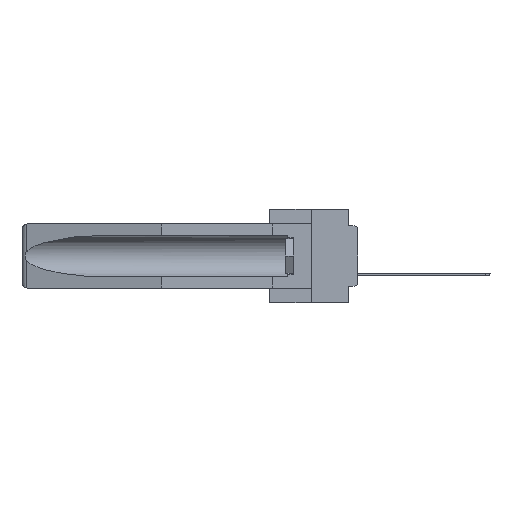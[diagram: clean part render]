
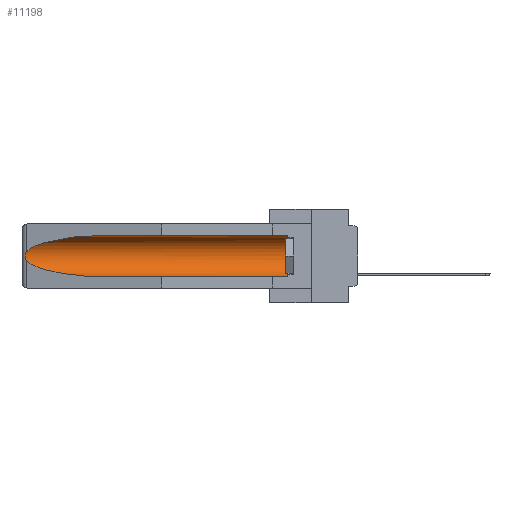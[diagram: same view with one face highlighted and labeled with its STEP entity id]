
A CAD part, left-side view. The second image highlights one B-rep face of the part: STEP entity #11198.
In plain terms, the highlighted cylindrical face has radius 2.857 mm (diameter 5.715 mm), a partial arc.
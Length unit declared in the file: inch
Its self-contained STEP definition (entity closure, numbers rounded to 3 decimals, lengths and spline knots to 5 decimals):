
#1793 = CIRCLE ( 'NONE', #25780, 0.1125 ) ;
#2804 = EDGE_CURVE ( 'NONE', #11947, #5407, #24546, .T. ) ;
#2918 = CARTESIAN_POINT ( 'NONE',  ( 0.26597, 1.52961, -0.15275 ) ) ;
#3536 = VECTOR ( 'NONE', #25333, 39.37008 ) ;
#3707 = CARTESIAN_POINT ( 'NONE',  ( 0.155, -0.30754, -0.1715 ) ) ;
#4063 = DIRECTION ( 'NONE',  ( 0., 1., 0. ) ) ;
#4702 = VERTEX_POINT ( 'NONE', #28749 ) ;
#5165 = VERTEX_POINT ( 'NONE', #16632 ) ;
#5407 = VERTEX_POINT ( 'NONE', #25781 ) ;
#5411 = CARTESIAN_POINT ( 'NONE',  ( 0.2675, 1.53308, -0.17534 ) ) ;
#5635 = CARTESIAN_POINT ( 'NONE',  ( 0.26597, 1.5296, -0.19026 ) ) ;
#5731 = CARTESIAN_POINT ( 'NONE',  ( 0.26537, 1.52718, -0.19328 ) ) ;
#7159 = LINE ( 'NONE', #12648, #3536 ) ;
#7700 = EDGE_CURVE ( 'NONE', #5165, #10313, #9998, .T. ) ;
#8202 = ORIENTED_EDGE ( 'NONE', *, *, #21001, .T. ) ;
#8883 = VECTOR ( 'NONE', #31061, 39.37008 ) ;
#9124 = AXIS2_PLACEMENT_3D ( 'NONE', #3707, #4063, #14493 ) ;
#9139 = CARTESIAN_POINT ( 'NONE',  ( 0.26537, 1.52718, -0.14972 ) ) ;
#9626 = EDGE_CURVE ( 'NONE', #10486, #11947, #1793, .T. ) ;
#9998 =( BOUNDED_CURVE ( )  B_SPLINE_CURVE ( 3, ( #27462, #22302, #32775, #30266 ),
 .UNSPECIFIED., .F., .F. ) 
 B_SPLINE_CURVE_WITH_KNOTS ( ( 4, 4 ),
 ( 0.1948, 1.5708 ),
 .UNSPECIFIED. ) 
 CURVE ( )  GEOMETRIC_REPRESENTATION_ITEM ( )  RATIONAL_B_SPLINE_CURVE ( ( 1., 0.848, 0.848, 1. ) ) 
 REPRESENTATION_ITEM ( '' )  );
#10286 = ORIENTED_EDGE ( 'NONE', *, *, #9626, .T. ) ;
#10313 = VERTEX_POINT ( 'NONE', #30845 ) ;
#10486 = VERTEX_POINT ( 'NONE', #29428 ) ;
#10651 = CARTESIAN_POINT ( 'NONE',  ( 0.2673, 1.53269, -0.17917 ) ) ;
#10661 = EDGE_LOOP ( 'NONE', ( #23231, #8202, #16517, #16245, #10286, #27308 ) ) ;
#10835 = FACE_OUTER_BOUND ( 'NONE', #10661, .T. ) ;
#11137 = CARTESIAN_POINT ( 'NONE',  ( 0.25451, 1.48313, -0.09465 ) ) ;
#11198 = ADVANCED_FACE ( 'NONE', ( #10835 ), #18476, .F. ) ;
#11947 = VERTEX_POINT ( 'NONE', #14923 ) ;
#12648 = CARTESIAN_POINT ( 'NONE',  ( 0.155, -0.30754, -0.284 ) ) ;
#13074 = CARTESIAN_POINT ( 'NONE',  ( 0.155, -0.30754, -0.059 ) ) ;
#14493 = DIRECTION ( 'NONE',  ( 0., 0., 1. ) ) ;
#14923 = CARTESIAN_POINT ( 'NONE',  ( 0.155, 0.126, -0.059 ) ) ;
#16245 = ORIENTED_EDGE ( 'NONE', *, *, #21391, .F. ) ;
#16517 = ORIENTED_EDGE ( 'NONE', *, *, #7700, .T. ) ;
#16632 = CARTESIAN_POINT ( 'NONE',  ( 0.26537, 1.52718, -0.19328 ) ) ;
#18269 = CARTESIAN_POINT ( 'NONE',  ( 0.26655, 1.53094, -0.18657 ) ) ;
#18476 = CYLINDRICAL_SURFACE ( 'NONE', #9124, 0.1125 ) ;
#18505 = CARTESIAN_POINT ( 'NONE',  ( 0.26654, 1.53092, -0.15636 ) ) ;
#19016 = B_SPLINE_CURVE_WITH_KNOTS ( 'NONE', 3,
 ( #31439, #2918, #18505, #28531, #21087, #5411, #10651, #18269, #5635, #5731 ),
 .UNSPECIFIED., .F., .F.,
 ( 4, 2, 2, 2, 4 ),
 ( 0., 0.00029, 0.00058, 0.00087, 0.00117 ),
 .UNSPECIFIED. ) ;
#21001 = EDGE_CURVE ( 'NONE', #4702, #5165, #19016, .T. ) ;
#21087 = CARTESIAN_POINT ( 'NONE',  ( 0.2675, 1.53308, -0.16763 ) ) ;
#21391 = EDGE_CURVE ( 'NONE', #10486, #10313, #7159, .T. ) ;
#21472 = CARTESIAN_POINT ( 'NONE',  ( 0.155, 1.07973, -0.059 ) ) ;
#22302 = CARTESIAN_POINT ( 'NONE',  ( 0.25451, 1.48313, -0.24835 ) ) ;
#23231 = ORIENTED_EDGE ( 'NONE', *, *, #29742, .T. ) ;
#24546 = LINE ( 'NONE', #13074, #8883 ) ;
#25333 = DIRECTION ( 'NONE',  ( 0., 1., 0. ) ) ;
#25780 = AXIS2_PLACEMENT_3D ( 'NONE', #28187, #27961, #30548 ) ;
#25781 = CARTESIAN_POINT ( 'NONE',  ( 0.155, 1.07973, -0.059 ) ) ;
#27308 = ORIENTED_EDGE ( 'NONE', *, *, #2804, .T. ) ;
#27462 = CARTESIAN_POINT ( 'NONE',  ( 0.26537, 1.52718, -0.19328 ) ) ;
#27961 = DIRECTION ( 'NONE',  ( 0., -1., 0. ) ) ;
#28187 = CARTESIAN_POINT ( 'NONE',  ( 0.155, 0.126, -0.1715 ) ) ;
#28531 = CARTESIAN_POINT ( 'NONE',  ( 0.2673, 1.5327, -0.16383 ) ) ;
#28686 = CARTESIAN_POINT ( 'NONE',  ( 0.21114, 1.30732, -0.059 ) ) ;
#28749 = CARTESIAN_POINT ( 'NONE',  ( 0.26537, 1.52718, -0.14972 ) ) ;
#29428 = CARTESIAN_POINT ( 'NONE',  ( 0.155, 0.126, -0.284 ) ) ;
#29520 =( BOUNDED_CURVE ( )  B_SPLINE_CURVE ( 3, ( #21472, #28686, #11137, #9139 ),
 .UNSPECIFIED., .F., .F. ) 
 B_SPLINE_CURVE_WITH_KNOTS ( ( 4, 4 ),
 ( 4.71239, 6.08839 ),
 .UNSPECIFIED. ) 
 CURVE ( )  GEOMETRIC_REPRESENTATION_ITEM ( )  RATIONAL_B_SPLINE_CURVE ( ( 1., 0.848, 0.848, 1. ) ) 
 REPRESENTATION_ITEM ( '' )  );
#29742 = EDGE_CURVE ( 'NONE', #5407, #4702, #29520, .T. ) ;
#30266 = CARTESIAN_POINT ( 'NONE',  ( 0.155, 1.07973, -0.284 ) ) ;
#30548 = DIRECTION ( 'NONE',  ( 0., 0., 1. ) ) ;
#30845 = CARTESIAN_POINT ( 'NONE',  ( 0.155, 1.07973, -0.284 ) ) ;
#31061 = DIRECTION ( 'NONE',  ( 0., 1., 0. ) ) ;
#31439 = CARTESIAN_POINT ( 'NONE',  ( 0.26537, 1.52718, -0.14972 ) ) ;
#32775 = CARTESIAN_POINT ( 'NONE',  ( 0.21114, 1.30732, -0.284 ) ) ;
